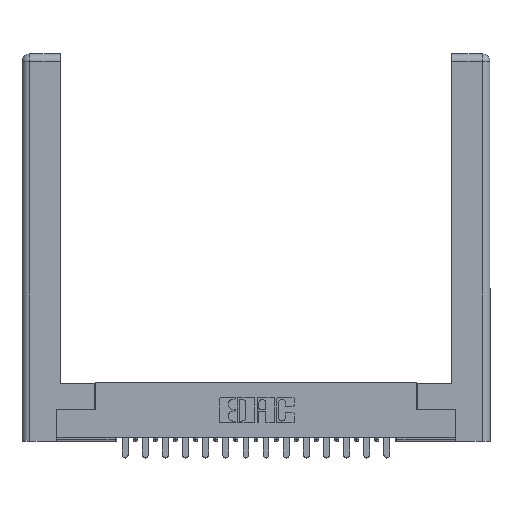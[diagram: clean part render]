
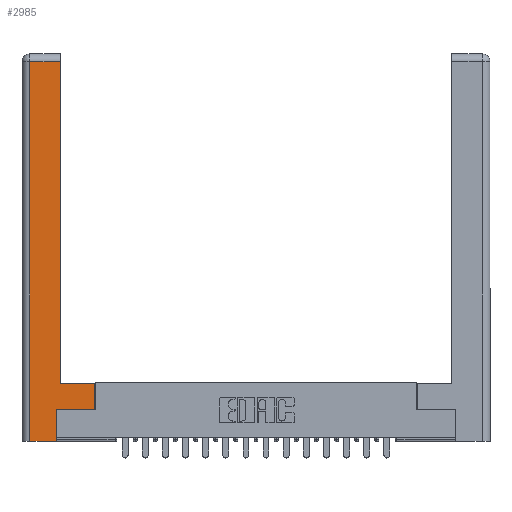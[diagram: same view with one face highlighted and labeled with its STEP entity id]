
A CAD part, top view. The second image highlights one B-rep face of the part: STEP entity #2985.
In plain terms, the highlighted planar face has unit normal (0, 0, 1).
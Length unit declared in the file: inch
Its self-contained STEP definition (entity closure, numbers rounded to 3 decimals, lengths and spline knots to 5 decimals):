
#38 = AXIS2_PLACEMENT_3D ( 'NONE', #20625, #14132, #4108 ) ;
#739 = CARTESIAN_POINT ( 'NONE',  ( 0.265, 0.245, 0. ) ) ;
#891 = VERTEX_POINT ( 'NONE', #12023 ) ;
#931 = EDGE_CURVE ( 'NONE', #20483, #7870, #1248, .T. ) ;
#1210 = EDGE_CURVE ( 'NONE', #891, #8857, #2006, .T. ) ;
#1248 = LINE ( 'NONE', #17051, #4054 ) ;
#1656 = DIRECTION ( 'NONE',  ( 1., 0., 0. ) ) ;
#1706 = EDGE_LOOP ( 'NONE', ( #13580, #4025, #19229, #11480, #14795, #20334, #9770, #9109 ) ) ;
#2006 = LINE ( 'NONE', #20308, #18834 ) ;
#2044 = CARTESIAN_POINT ( 'NONE',  ( 0.265, 0., 0. ) ) ;
#2368 = EDGE_CURVE ( 'NONE', #14075, #891, #12160, .T. ) ;
#2598 = LINE ( 'NONE', #6452, #4632 ) ;
#2985 = ADVANCED_FACE ( 'NONE', ( #5233 ), #9150, .F. ) ;
#4025 = ORIENTED_EDGE ( 'NONE', *, *, #931, .T. ) ;
#4054 = VECTOR ( 'NONE', #7323, 39.37008 ) ;
#4108 = DIRECTION ( 'NONE',  ( -1., 0., 0. ) ) ;
#4174 = EDGE_CURVE ( 'NONE', #11217, #14075, #2598, .T. ) ;
#4473 = VECTOR ( 'NONE', #5166, 39.37008 ) ;
#4632 = VECTOR ( 'NONE', #19770, 39.37008 ) ;
#5166 = DIRECTION ( 'NONE',  ( -1., 0., 0. ) ) ;
#5233 = FACE_OUTER_BOUND ( 'NONE', #1706, .T. ) ;
#6188 = VERTEX_POINT ( 'NONE', #13760 ) ;
#6301 = DIRECTION ( 'NONE',  ( 0., 1., 0. ) ) ;
#6330 = EDGE_CURVE ( 'NONE', #17553, #11217, #11717, .T. ) ;
#6452 = CARTESIAN_POINT ( 'NONE',  ( 0.265, 0.245, 0. ) ) ;
#6550 = CARTESIAN_POINT ( 'NONE',  ( 0.565, 0.45, 0. ) ) ;
#7323 = DIRECTION ( 'NONE',  ( -1., 0., 0. ) ) ;
#7805 = VECTOR ( 'NONE', #15301, 39.37008 ) ;
#7870 = VERTEX_POINT ( 'NONE', #17258 ) ;
#8138 = VECTOR ( 'NONE', #15511, 39.37008 ) ;
#8149 = EDGE_CURVE ( 'NONE', #8857, #6188, #20792, .T. ) ;
#8301 = CARTESIAN_POINT ( 'NONE',  ( 0.0615, 0., 0. ) ) ;
#8702 = DIRECTION ( 'NONE',  ( 0., 1., 0. ) ) ;
#8857 = VERTEX_POINT ( 'NONE', #6550 ) ;
#9109 = ORIENTED_EDGE ( 'NONE', *, *, #8149, .T. ) ;
#9150 = PLANE ( 'NONE',  #38 ) ;
#9770 = ORIENTED_EDGE ( 'NONE', *, *, #1210, .T. ) ;
#9995 = CARTESIAN_POINT ( 'NONE',  ( 0.295, 0.45, 0. ) ) ;
#10423 = CARTESIAN_POINT ( 'NONE',  ( 0.0615, 0., 0. ) ) ;
#10852 = LINE ( 'NONE', #21100, #16901 ) ;
#11217 = VERTEX_POINT ( 'NONE', #2044 ) ;
#11480 = ORIENTED_EDGE ( 'NONE', *, *, #6330, .T. ) ;
#11717 = LINE ( 'NONE', #12132, #8138 ) ;
#12023 = CARTESIAN_POINT ( 'NONE',  ( 0.565, 0.245, 0. ) ) ;
#12132 = CARTESIAN_POINT ( 'NONE',  ( 0.265, 0., 0. ) ) ;
#12160 = LINE ( 'NONE', #14799, #16198 ) ;
#13530 = EDGE_CURVE ( 'NONE', #7870, #17553, #20271, .T. ) ;
#13580 = ORIENTED_EDGE ( 'NONE', *, *, #20995, .T. ) ;
#13760 = CARTESIAN_POINT ( 'NONE',  ( 0.295, 0.45, 0. ) ) ;
#14075 = VERTEX_POINT ( 'NONE', #739 ) ;
#14132 = DIRECTION ( 'NONE',  ( 0., 0., -1. ) ) ;
#14795 = ORIENTED_EDGE ( 'NONE', *, *, #4174, .T. ) ;
#14799 = CARTESIAN_POINT ( 'NONE',  ( 0.565, 0.245, 0. ) ) ;
#15301 = DIRECTION ( 'NONE',  ( 0., -1., 0. ) ) ;
#15511 = DIRECTION ( 'NONE',  ( 1., 0., 0. ) ) ;
#16198 = VECTOR ( 'NONE', #1656, 39.37008 ) ;
#16901 = VECTOR ( 'NONE', #6301, 39.37008 ) ;
#17051 = CARTESIAN_POINT ( 'NONE',  ( 0.0615, 2.94, 0. ) ) ;
#17258 = CARTESIAN_POINT ( 'NONE',  ( 0.0615, 2.94, 0. ) ) ;
#17553 = VERTEX_POINT ( 'NONE', #8301 ) ;
#18834 = VECTOR ( 'NONE', #8702, 39.37008 ) ;
#19229 = ORIENTED_EDGE ( 'NONE', *, *, #13530, .T. ) ;
#19717 = CARTESIAN_POINT ( 'NONE',  ( 0.295, 2.94, 0. ) ) ;
#19770 = DIRECTION ( 'NONE',  ( 0., 1., 0. ) ) ;
#20271 = LINE ( 'NONE', #10423, #7805 ) ;
#20308 = CARTESIAN_POINT ( 'NONE',  ( 0.565, 0.45, 0. ) ) ;
#20334 = ORIENTED_EDGE ( 'NONE', *, *, #2368, .T. ) ;
#20483 = VERTEX_POINT ( 'NONE', #19717 ) ;
#20625 = CARTESIAN_POINT ( 'NONE',  ( 0., 0., 0. ) ) ;
#20792 = LINE ( 'NONE', #9995, #4473 ) ;
#20995 = EDGE_CURVE ( 'NONE', #6188, #20483, #10852, .T. ) ;
#21100 = CARTESIAN_POINT ( 'NONE',  ( 0.295, 3., 0. ) ) ;
